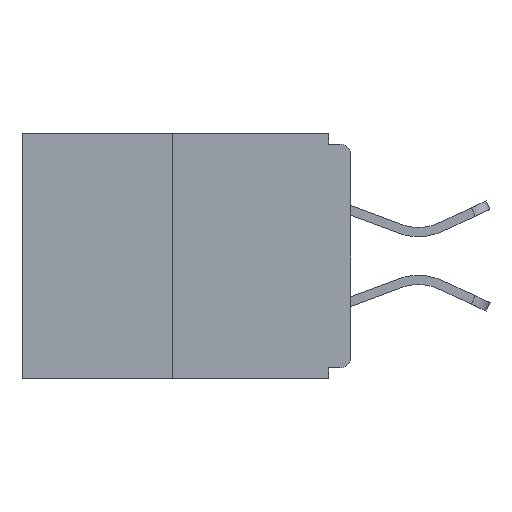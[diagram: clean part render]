
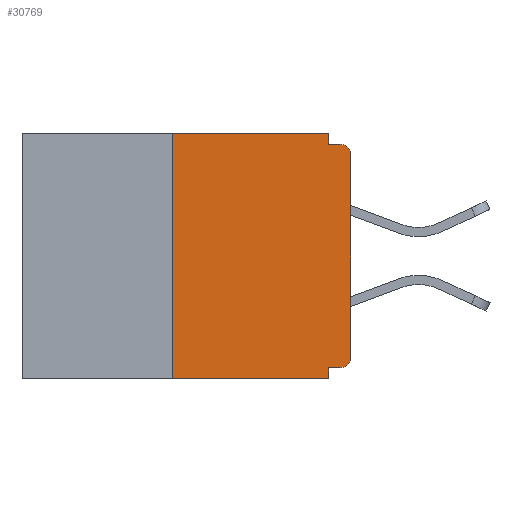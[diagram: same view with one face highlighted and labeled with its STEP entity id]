
A CAD part, left-side view. The second image highlights one B-rep face of the part: STEP entity #30769.
In plain terms, the highlighted planar face has unit normal (-1, 0, 0).
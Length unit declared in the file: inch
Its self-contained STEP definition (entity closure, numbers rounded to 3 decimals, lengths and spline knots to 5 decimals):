
#138 = LINE ( 'NONE', #14938, #22459 ) ;
#396 = EDGE_CURVE ( 'NONE', #4376, #17863, #7089, .T. ) ;
#979 = EDGE_CURVE ( 'NONE', #20302, #21963, #10563, .T. ) ;
#1110 = CARTESIAN_POINT ( 'NONE',  ( 0., 0.031, -0.328 ) ) ;
#1626 = EDGE_CURVE ( 'NONE', #14669, #3183, #31195, .T. ) ;
#1857 = CARTESIAN_POINT ( 'NONE',  ( 0., 0.031, 0. ) ) ;
#1866 = VERTEX_POINT ( 'NONE', #10176 ) ;
#2311 = VECTOR ( 'NONE', #19864, 39.37008 ) ;
#2661 = VECTOR ( 'NONE', #8203, 39.37008 ) ;
#2703 = FACE_OUTER_BOUND ( 'NONE', #23678, .T. ) ;
#3183 = VERTEX_POINT ( 'NONE', #7976 ) ;
#3556 = EDGE_CURVE ( 'NONE', #12776, #4376, #21599, .T. ) ;
#3947 = DIRECTION ( 'NONE',  ( 0., 0., -1. ) ) ;
#4061 = EDGE_CURVE ( 'NONE', #21963, #8452, #16450, .T. ) ;
#4376 = VERTEX_POINT ( 'NONE', #13047 ) ;
#4646 = DIRECTION ( 'NONE',  ( 0., 0., -1. ) ) ;
#4997 = DIRECTION ( 'NONE',  ( 0., 0., -1. ) ) ;
#5957 = DIRECTION ( 'NONE',  ( 0., 0., -1. ) ) ;
#6197 = CARTESIAN_POINT ( 'NONE',  ( 0., 0., 0. ) ) ;
#6338 = VECTOR ( 'NONE', #28784, 39.37008 ) ;
#6905 = CARTESIAN_POINT ( 'NONE',  ( 0., 0.46, 0. ) ) ;
#7089 = LINE ( 'NONE', #14925, #15194 ) ;
#7955 = AXIS2_PLACEMENT_3D ( 'NONE', #29070, #16561, #4997 ) ;
#7976 = CARTESIAN_POINT ( 'NONE',  ( 0., 0., -0.03 ) ) ;
#8021 = AXIS2_PLACEMENT_3D ( 'NONE', #15424, #8040, #5957 ) ;
#8040 = DIRECTION ( 'NONE',  ( -1., 0., 0. ) ) ;
#8203 = DIRECTION ( 'NONE',  ( 0., -1., 0. ) ) ;
#8452 = VERTEX_POINT ( 'NONE', #29673 ) ;
#8618 = ORIENTED_EDGE ( 'NONE', *, *, #3556, .F. ) ;
#10076 = CARTESIAN_POINT ( 'NONE',  ( 0., 0., -0.328 ) ) ;
#10176 = CARTESIAN_POINT ( 'NONE',  ( 0., 0.25, -0.343 ) ) ;
#10450 = ORIENTED_EDGE ( 'NONE', *, *, #11811, .T. ) ;
#10563 = LINE ( 'NONE', #10076, #2311 ) ;
#11357 = DIRECTION ( 'NONE',  ( 0., 0., -1. ) ) ;
#11811 = EDGE_CURVE ( 'NONE', #3183, #17863, #14104, .T. ) ;
#12504 = PLANE ( 'NONE',  #13668 ) ;
#12600 = VECTOR ( 'NONE', #21594, 39.37008 ) ;
#12776 = VERTEX_POINT ( 'NONE', #20451 ) ;
#12853 = ORIENTED_EDGE ( 'NONE', *, *, #31634, .T. ) ;
#13018 = CARTESIAN_POINT ( 'NONE',  ( 0., 0.46, -0.343 ) ) ;
#13047 = CARTESIAN_POINT ( 'NONE',  ( 0., 0.031, -0.015 ) ) ;
#13133 = ORIENTED_EDGE ( 'NONE', *, *, #979, .F. ) ;
#13339 = ORIENTED_EDGE ( 'NONE', *, *, #14859, .F. ) ;
#13668 = AXIS2_PLACEMENT_3D ( 'NONE', #6905, #14762, #4646 ) ;
#14104 = CIRCLE ( 'NONE', #7955, 0.015 ) ;
#14669 = VERTEX_POINT ( 'NONE', #18644 ) ;
#14762 = DIRECTION ( 'NONE',  ( 1., 0., 0. ) ) ;
#14859 = EDGE_CURVE ( 'NONE', #16268, #12776, #138, .T. ) ;
#14925 = CARTESIAN_POINT ( 'NONE',  ( 0., 0., -0.015 ) ) ;
#14938 = CARTESIAN_POINT ( 'NONE',  ( 0., 0.46, 0. ) ) ;
#15194 = VECTOR ( 'NONE', #31288, 39.37008 ) ;
#15424 = CARTESIAN_POINT ( 'NONE',  ( 0., 0.015, -0.313 ) ) ;
#16268 = VERTEX_POINT ( 'NONE', #22868 ) ;
#16450 = LINE ( 'NONE', #19128, #31523 ) ;
#16561 = DIRECTION ( 'NONE',  ( -1., 0., 0. ) ) ;
#17863 = VERTEX_POINT ( 'NONE', #25708 ) ;
#18644 = CARTESIAN_POINT ( 'NONE',  ( 0., 0., -0.313 ) ) ;
#19000 = EDGE_CURVE ( 'NONE', #1866, #16268, #28966, .T. ) ;
#19128 = CARTESIAN_POINT ( 'NONE',  ( 0., 0.031, -0.343 ) ) ;
#19864 = DIRECTION ( 'NONE',  ( 0., 1., 0. ) ) ;
#20302 = VERTEX_POINT ( 'NONE', #23547 ) ;
#20451 = CARTESIAN_POINT ( 'NONE',  ( 0., 0.031, 0. ) ) ;
#21037 = ORIENTED_EDGE ( 'NONE', *, *, #19000, .F. ) ;
#21359 = CIRCLE ( 'NONE', #8021, 0.015 ) ;
#21594 = DIRECTION ( 'NONE',  ( 0., 0., 1. ) ) ;
#21599 = LINE ( 'NONE', #1857, #31077 ) ;
#21963 = VERTEX_POINT ( 'NONE', #1110 ) ;
#22056 = CARTESIAN_POINT ( 'NONE',  ( 0., 0.25, 0. ) ) ;
#22459 = VECTOR ( 'NONE', #24714, 39.37008 ) ;
#22511 = ORIENTED_EDGE ( 'NONE', *, *, #4061, .F. ) ;
#22632 = ORIENTED_EDGE ( 'NONE', *, *, #1626, .T. ) ;
#22868 = CARTESIAN_POINT ( 'NONE',  ( 0., 0.25, 0. ) ) ;
#23120 = EDGE_CURVE ( 'NONE', #1866, #8452, #27608, .T. ) ;
#23547 = CARTESIAN_POINT ( 'NONE',  ( 0., 0.015, -0.328 ) ) ;
#23678 = EDGE_LOOP ( 'NONE', ( #13339, #21037, #25576, #22511, #13133, #12853, #22632, #10450, #25038, #8618 ) ) ;
#24714 = DIRECTION ( 'NONE',  ( 0., -1., 0. ) ) ;
#25038 = ORIENTED_EDGE ( 'NONE', *, *, #396, .F. ) ;
#25576 = ORIENTED_EDGE ( 'NONE', *, *, #23120, .T. ) ;
#25708 = CARTESIAN_POINT ( 'NONE',  ( 0., 0.015, -0.015 ) ) ;
#27608 = LINE ( 'NONE', #13018, #2661 ) ;
#28784 = DIRECTION ( 'NONE',  ( 0., 0., 1. ) ) ;
#28966 = LINE ( 'NONE', #22056, #12600 ) ;
#29070 = CARTESIAN_POINT ( 'NONE',  ( 0., 0.015, -0.03 ) ) ;
#29673 = CARTESIAN_POINT ( 'NONE',  ( 0., 0.031, -0.343 ) ) ;
#30769 = ADVANCED_FACE ( 'NONE', ( #2703 ), #12504, .F. ) ;
#31077 = VECTOR ( 'NONE', #11357, 39.37008 ) ;
#31195 = LINE ( 'NONE', #6197, #6338 ) ;
#31288 = DIRECTION ( 'NONE',  ( 0., -1., 0. ) ) ;
#31523 = VECTOR ( 'NONE', #3947, 39.37008 ) ;
#31634 = EDGE_CURVE ( 'NONE', #20302, #14669, #21359, .T. ) ;
